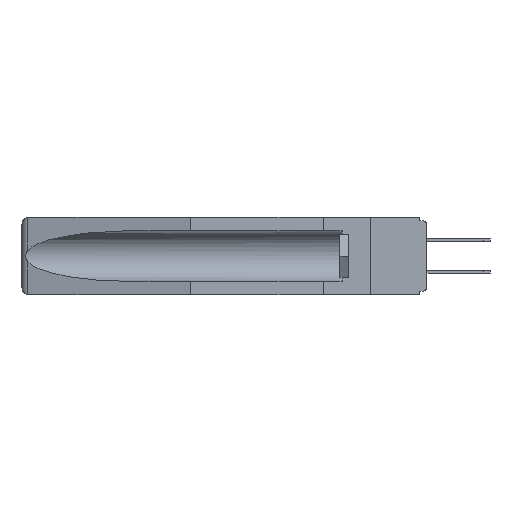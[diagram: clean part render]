
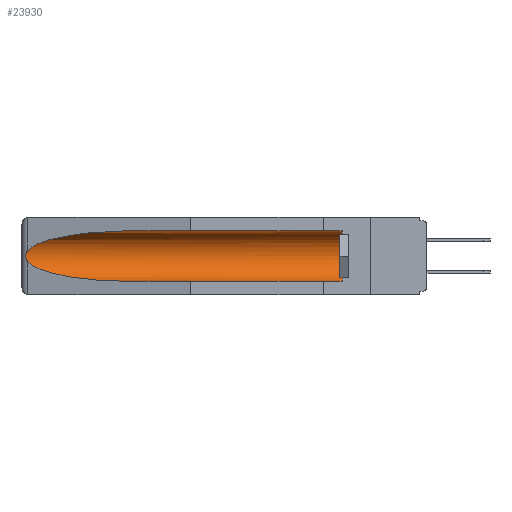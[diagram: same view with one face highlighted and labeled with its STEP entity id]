
A CAD part, left-side view. The second image highlights one B-rep face of the part: STEP entity #23930.
In plain terms, the highlighted cylindrical face has radius 2.857 mm (diameter 5.715 mm), a partial arc.
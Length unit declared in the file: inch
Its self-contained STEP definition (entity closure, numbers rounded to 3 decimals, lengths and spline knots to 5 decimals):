
#917 = VERTEX_POINT ( 'NONE', #15719 ) ;
#1266 = CYLINDRICAL_SURFACE ( 'NONE', #13797, 0.1125 ) ;
#1287 = FACE_OUTER_BOUND ( 'NONE', #7877, .T. ) ;
#1477 = DIRECTION ( 'NONE',  ( 0., 0., 1. ) ) ;
#1864 =( BOUNDED_CURVE ( )  B_SPLINE_CURVE ( 3, ( #10023, #19495, #11894, #13936 ),
 .UNSPECIFIED., .F., .F. ) 
 B_SPLINE_CURVE_WITH_KNOTS ( ( 4, 4 ),
 ( 4.71239, 6.08839 ),
 .UNSPECIFIED. ) 
 CURVE ( )  GEOMETRIC_REPRESENTATION_ITEM ( )  RATIONAL_B_SPLINE_CURVE ( ( 1., 0.848, 0.848, 1. ) ) 
 REPRESENTATION_ITEM ( '' )  );
#2107 = ORIENTED_EDGE ( 'NONE', *, *, #2531, .T. ) ;
#2531 = EDGE_CURVE ( 'NONE', #22671, #17519, #8252, .T. ) ;
#2843 = CARTESIAN_POINT ( 'NONE',  ( 0.2673, 1.5327, -0.16383 ) ) ;
#2921 = CARTESIAN_POINT ( 'NONE',  ( 0.2673, 1.53269, -0.17917 ) ) ;
#2990 = EDGE_CURVE ( 'NONE', #3305, #917, #4023, .T. ) ;
#3305 = VERTEX_POINT ( 'NONE', #10893 ) ;
#4023 = LINE ( 'NONE', #21961, #9520 ) ;
#4129 = DIRECTION ( 'NONE',  ( 0., 1., 0. ) ) ;
#4369 = ORIENTED_EDGE ( 'NONE', *, *, #12955, .T. ) ;
#5229 = DIRECTION ( 'NONE',  ( 0., -1., 0. ) ) ;
#6082 = EDGE_CURVE ( 'NONE', #6564, #11957, #9388, .T. ) ;
#6225 = VECTOR ( 'NONE', #4129, 39.37008 ) ;
#6451 =( BOUNDED_CURVE ( )  B_SPLINE_CURVE ( 3, ( #9954, #11919, #7223, #19968 ),
 .UNSPECIFIED., .F., .F. ) 
 B_SPLINE_CURVE_WITH_KNOTS ( ( 4, 4 ),
 ( 0.1948, 1.5708 ),
 .UNSPECIFIED. ) 
 CURVE ( )  GEOMETRIC_REPRESENTATION_ITEM ( )  RATIONAL_B_SPLINE_CURVE ( ( 1., 0.848, 0.848, 1. ) ) 
 REPRESENTATION_ITEM ( '' )  );
#6564 = VERTEX_POINT ( 'NONE', #18516 ) ;
#6812 = CARTESIAN_POINT ( 'NONE',  ( 0.26537, 1.52718, -0.14972 ) ) ;
#6889 = CARTESIAN_POINT ( 'NONE',  ( 0.155, 1.07973, -0.284 ) ) ;
#7223 = CARTESIAN_POINT ( 'NONE',  ( 0.21114, 1.30732, -0.284 ) ) ;
#7877 = EDGE_LOOP ( 'NONE', ( #17779, #2107, #4369, #16108, #9500, #16650 ) ) ;
#8252 = B_SPLINE_CURVE_WITH_KNOTS ( 'NONE', 3,
 ( #15641, #23054, #23123, #2843, #10263, #23198, #2921, #15881, #10348, #23285 ),
 .UNSPECIFIED., .F., .F.,
 ( 4, 2, 2, 2, 4 ),
 ( 0., 0.00029, 0.00058, 0.00087, 0.00117 ),
 .UNSPECIFIED. ) ;
#8609 = DIRECTION ( 'NONE',  ( 0., 1., 0. ) ) ;
#9179 = DIRECTION ( 'NONE',  ( 0., 1., 0. ) ) ;
#9388 = LINE ( 'NONE', #13294, #6225 ) ;
#9500 = ORIENTED_EDGE ( 'NONE', *, *, #17322, .T. ) ;
#9520 = VECTOR ( 'NONE', #9179, 39.37008 ) ;
#9954 = CARTESIAN_POINT ( 'NONE',  ( 0.26537, 1.52718, -0.19328 ) ) ;
#10023 = CARTESIAN_POINT ( 'NONE',  ( 0.155, 1.07973, -0.059 ) ) ;
#10263 = CARTESIAN_POINT ( 'NONE',  ( 0.2675, 1.53308, -0.16763 ) ) ;
#10348 = CARTESIAN_POINT ( 'NONE',  ( 0.26597, 1.5296, -0.19026 ) ) ;
#10893 = CARTESIAN_POINT ( 'NONE',  ( 0.155, 0.126, -0.059 ) ) ;
#10997 = DIRECTION ( 'NONE',  ( 0., 0., 1. ) ) ;
#11894 = CARTESIAN_POINT ( 'NONE',  ( 0.25451, 1.48313, -0.09465 ) ) ;
#11919 = CARTESIAN_POINT ( 'NONE',  ( 0.25451, 1.48313, -0.24835 ) ) ;
#11957 = VERTEX_POINT ( 'NONE', #6889 ) ;
#12955 = EDGE_CURVE ( 'NONE', #17519, #11957, #6451, .T. ) ;
#13294 = CARTESIAN_POINT ( 'NONE',  ( 0.155, -0.30754, -0.284 ) ) ;
#13354 = AXIS2_PLACEMENT_3D ( 'NONE', #16516, #5229, #10997 ) ;
#13797 = AXIS2_PLACEMENT_3D ( 'NONE', #14129, #8609, #1477 ) ;
#13936 = CARTESIAN_POINT ( 'NONE',  ( 0.26537, 1.52718, -0.14972 ) ) ;
#14129 = CARTESIAN_POINT ( 'NONE',  ( 0.155, -0.30754, -0.1715 ) ) ;
#15641 = CARTESIAN_POINT ( 'NONE',  ( 0.26537, 1.52718, -0.14972 ) ) ;
#15719 = CARTESIAN_POINT ( 'NONE',  ( 0.155, 1.07973, -0.059 ) ) ;
#15881 = CARTESIAN_POINT ( 'NONE',  ( 0.26655, 1.53094, -0.18657 ) ) ;
#16108 = ORIENTED_EDGE ( 'NONE', *, *, #6082, .F. ) ;
#16516 = CARTESIAN_POINT ( 'NONE',  ( 0.155, 0.126, -0.1715 ) ) ;
#16650 = ORIENTED_EDGE ( 'NONE', *, *, #2990, .T. ) ;
#17138 = EDGE_CURVE ( 'NONE', #917, #22671, #1864, .T. ) ;
#17322 = EDGE_CURVE ( 'NONE', #6564, #3305, #20884, .T. ) ;
#17519 = VERTEX_POINT ( 'NONE', #22128 ) ;
#17779 = ORIENTED_EDGE ( 'NONE', *, *, #17138, .T. ) ;
#18516 = CARTESIAN_POINT ( 'NONE',  ( 0.155, 0.126, -0.284 ) ) ;
#19495 = CARTESIAN_POINT ( 'NONE',  ( 0.21114, 1.30732, -0.059 ) ) ;
#19968 = CARTESIAN_POINT ( 'NONE',  ( 0.155, 1.07973, -0.284 ) ) ;
#20884 = CIRCLE ( 'NONE', #13354, 0.1125 ) ;
#21961 = CARTESIAN_POINT ( 'NONE',  ( 0.155, -0.30754, -0.059 ) ) ;
#22128 = CARTESIAN_POINT ( 'NONE',  ( 0.26537, 1.52718, -0.19328 ) ) ;
#22671 = VERTEX_POINT ( 'NONE', #6812 ) ;
#23054 = CARTESIAN_POINT ( 'NONE',  ( 0.26597, 1.52961, -0.15275 ) ) ;
#23123 = CARTESIAN_POINT ( 'NONE',  ( 0.26654, 1.53092, -0.15636 ) ) ;
#23198 = CARTESIAN_POINT ( 'NONE',  ( 0.2675, 1.53308, -0.17534 ) ) ;
#23285 = CARTESIAN_POINT ( 'NONE',  ( 0.26537, 1.52718, -0.19328 ) ) ;
#23930 = ADVANCED_FACE ( 'NONE', ( #1287 ), #1266, .F. ) ;
